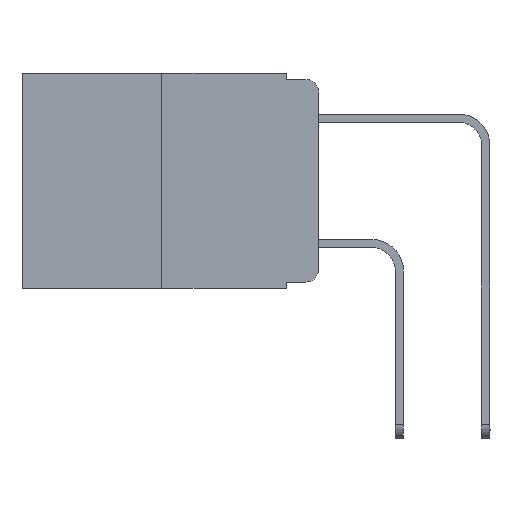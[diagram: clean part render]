
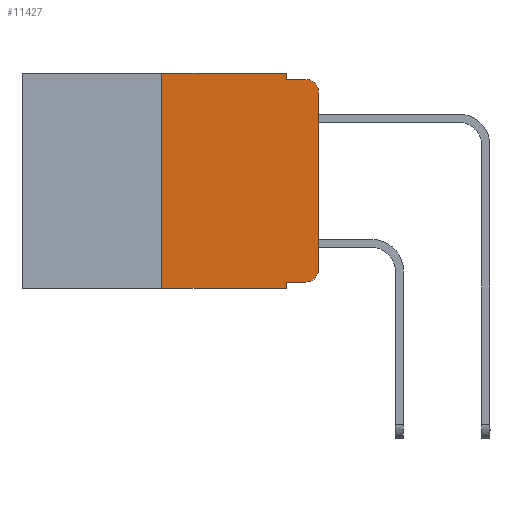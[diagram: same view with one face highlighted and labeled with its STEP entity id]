
A CAD part, left-side view. The second image highlights one B-rep face of the part: STEP entity #11427.
In plain terms, the highlighted planar face has unit normal (-1, 0, 0).
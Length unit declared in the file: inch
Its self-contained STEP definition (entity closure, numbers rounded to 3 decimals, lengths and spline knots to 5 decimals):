
#156 = VERTEX_POINT ( 'NONE', #11077 ) ;
#227 = CARTESIAN_POINT ( 'NONE',  ( 0., 0.473, 0. ) ) ;
#352 = CARTESIAN_POINT ( 'NONE',  ( 0., 0.25, -0.343 ) ) ;
#444 = CARTESIAN_POINT ( 'NONE',  ( 0., 0., 0. ) ) ;
#449 = DIRECTION ( 'NONE',  ( 0., -1., 0. ) ) ;
#507 = CARTESIAN_POINT ( 'NONE',  ( 0., 0.02, -0.313 ) ) ;
#919 = EDGE_CURVE ( 'NONE', #6880, #9221, #7108, .T. ) ;
#986 = LINE ( 'NONE', #4742, #7120 ) ;
#1049 = CIRCLE ( 'NONE', #4348, 0.02 ) ;
#1282 = CARTESIAN_POINT ( 'NONE',  ( 0., 0.25, 0. ) ) ;
#1283 = CARTESIAN_POINT ( 'NONE',  ( 0., 0.051, -0.333 ) ) ;
#1391 = AXIS2_PLACEMENT_3D ( 'NONE', #1422, #8281, #12203 ) ;
#1409 = CARTESIAN_POINT ( 'NONE',  ( 0., 0.051, -0.343 ) ) ;
#1422 = CARTESIAN_POINT ( 'NONE',  ( 0., 0.473, 0. ) ) ;
#1708 = VERTEX_POINT ( 'NONE', #5557 ) ;
#1714 = VERTEX_POINT ( 'NONE', #1409 ) ;
#2047 = DIRECTION ( 'NONE',  ( 0., -1., 0. ) ) ;
#2217 = PLANE ( 'NONE',  #1391 ) ;
#2336 = FACE_OUTER_BOUND ( 'NONE', #8867, .T. ) ;
#2341 = CARTESIAN_POINT ( 'NONE',  ( 0., 0.473, -0.343 ) ) ;
#2403 = ORIENTED_EDGE ( 'NONE', *, *, #8755, .F. ) ;
#2463 = DIRECTION ( 'NONE',  ( -1., 0., 0. ) ) ;
#2482 = VERTEX_POINT ( 'NONE', #10012 ) ;
#2637 = ORIENTED_EDGE ( 'NONE', *, *, #11166, .F. ) ;
#2876 = DIRECTION ( 'NONE',  ( 0., 0., 1. ) ) ;
#2899 = DIRECTION ( 'NONE',  ( 0., -1., 0. ) ) ;
#2945 = ORIENTED_EDGE ( 'NONE', *, *, #10287, .T. ) ;
#3021 = CARTESIAN_POINT ( 'NONE',  ( 0., 0.051, -0.01 ) ) ;
#3041 = VECTOR ( 'NONE', #2047, 39.37008 ) ;
#3043 = EDGE_CURVE ( 'NONE', #2482, #1708, #1049, .T. ) ;
#3325 = DIRECTION ( 'NONE',  ( 0., -1., 0. ) ) ;
#3717 = EDGE_CURVE ( 'NONE', #4159, #11202, #8184, .T. ) ;
#3983 = LINE ( 'NONE', #3021, #7406 ) ;
#4134 = VECTOR ( 'NONE', #3325, 39.37008 ) ;
#4159 = VERTEX_POINT ( 'NONE', #1282 ) ;
#4348 = AXIS2_PLACEMENT_3D ( 'NONE', #507, #2463, #7631 ) ;
#4547 = EDGE_CURVE ( 'NONE', #8547, #1714, #11310, .T. ) ;
#4611 = LINE ( 'NONE', #8553, #8404 ) ;
#4742 = CARTESIAN_POINT ( 'NONE',  ( 0., 0.25, 0. ) ) ;
#5015 = ORIENTED_EDGE ( 'NONE', *, *, #5180, .F. ) ;
#5180 = EDGE_CURVE ( 'NONE', #156, #9221, #3983, .T. ) ;
#5366 = LINE ( 'NONE', #444, #7144 ) ;
#5557 = CARTESIAN_POINT ( 'NONE',  ( 0., 0., -0.313 ) ) ;
#5589 = LINE ( 'NONE', #9507, #10662 ) ;
#5743 = CARTESIAN_POINT ( 'NONE',  ( 0., 0., -0.03 ) ) ;
#5779 = EDGE_CURVE ( 'NONE', #7540, #2482, #11902, .T. ) ;
#5784 = DIRECTION ( 'NONE',  ( 0., 0., -1. ) ) ;
#6005 = CARTESIAN_POINT ( 'NONE',  ( 0., 0.02, -0.01 ) ) ;
#6131 = ORIENTED_EDGE ( 'NONE', *, *, #919, .T. ) ;
#6880 = VERTEX_POINT ( 'NONE', #5743 ) ;
#7108 = CIRCLE ( 'NONE', #10602, 0.02 ) ;
#7120 = VECTOR ( 'NONE', #2876, 39.37008 ) ;
#7144 = VECTOR ( 'NONE', #10189, 39.37008 ) ;
#7406 = VECTOR ( 'NONE', #2899, 39.37008 ) ;
#7540 = VERTEX_POINT ( 'NONE', #1283 ) ;
#7631 = DIRECTION ( 'NONE',  ( 0., 0., -1. ) ) ;
#7656 = CARTESIAN_POINT ( 'NONE',  ( 0., 0.051, 0. ) ) ;
#7940 = ORIENTED_EDGE ( 'NONE', *, *, #4547, .T. ) ;
#7971 = DIRECTION ( 'NONE',  ( -1., 0., 0. ) ) ;
#8137 = VECTOR ( 'NONE', #449, 39.37008 ) ;
#8170 = ORIENTED_EDGE ( 'NONE', *, *, #3717, .F. ) ;
#8184 = LINE ( 'NONE', #227, #3041 ) ;
#8281 = DIRECTION ( 'NONE',  ( 1., 0., 0. ) ) ;
#8404 = VECTOR ( 'NONE', #5784, 39.37008 ) ;
#8547 = VERTEX_POINT ( 'NONE', #352 ) ;
#8553 = CARTESIAN_POINT ( 'NONE',  ( 0., 0.051, 0. ) ) ;
#8755 = EDGE_CURVE ( 'NONE', #8547, #4159, #986, .T. ) ;
#8867 = EDGE_LOOP ( 'NONE', ( #2945, #6131, #5015, #9345, #8170, #2403, #7940, #2637, #9900, #9307 ) ) ;
#9221 = VERTEX_POINT ( 'NONE', #6005 ) ;
#9307 = ORIENTED_EDGE ( 'NONE', *, *, #3043, .T. ) ;
#9345 = ORIENTED_EDGE ( 'NONE', *, *, #11237, .F. ) ;
#9507 = CARTESIAN_POINT ( 'NONE',  ( 0., 0.051, 0. ) ) ;
#9900 = ORIENTED_EDGE ( 'NONE', *, *, #5779, .T. ) ;
#9942 = CARTESIAN_POINT ( 'NONE',  ( 0., 0.02, -0.03 ) ) ;
#10012 = CARTESIAN_POINT ( 'NONE',  ( 0., 0.02, -0.333 ) ) ;
#10189 = DIRECTION ( 'NONE',  ( 0., 0., 1. ) ) ;
#10287 = EDGE_CURVE ( 'NONE', #1708, #6880, #5366, .T. ) ;
#10602 = AXIS2_PLACEMENT_3D ( 'NONE', #9942, #7971, #10855 ) ;
#10662 = VECTOR ( 'NONE', #10975, 39.37008 ) ;
#10855 = DIRECTION ( 'NONE',  ( 0., 0., -1. ) ) ;
#10975 = DIRECTION ( 'NONE',  ( 0., 0., -1. ) ) ;
#11077 = CARTESIAN_POINT ( 'NONE',  ( 0., 0.051, -0.01 ) ) ;
#11166 = EDGE_CURVE ( 'NONE', #7540, #1714, #4611, .T. ) ;
#11202 = VERTEX_POINT ( 'NONE', #7656 ) ;
#11237 = EDGE_CURVE ( 'NONE', #11202, #156, #5589, .T. ) ;
#11310 = LINE ( 'NONE', #2341, #8137 ) ;
#11427 = ADVANCED_FACE ( 'NONE', ( #2336 ), #2217, .F. ) ;
#11902 = LINE ( 'NONE', #12156, #4134 ) ;
#12156 = CARTESIAN_POINT ( 'NONE',  ( 0., 0.051, -0.333 ) ) ;
#12203 = DIRECTION ( 'NONE',  ( 0., 0., -1. ) ) ;
